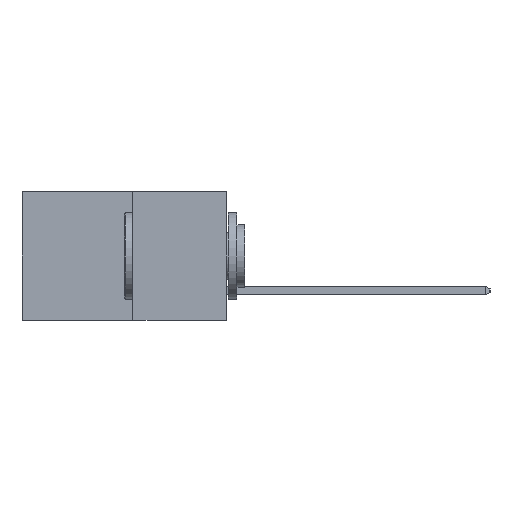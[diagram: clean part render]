
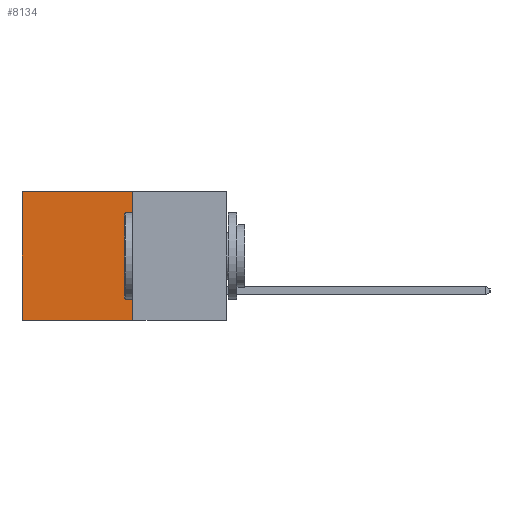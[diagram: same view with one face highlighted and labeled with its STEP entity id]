
A CAD part, left-side view. The second image highlights one B-rep face of the part: STEP entity #8134.
In plain terms, the highlighted planar face has unit normal (-1, 0, 0).
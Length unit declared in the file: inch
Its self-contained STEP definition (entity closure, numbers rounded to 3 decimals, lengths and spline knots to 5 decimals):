
#616 = PLANE ( 'NONE',  #6186 ) ;
#659 = EDGE_CURVE ( 'NONE', #6049, #8187, #4070, .T. ) ;
#682 = CARTESIAN_POINT ( 'NONE',  ( 0.277, 0.59, 0. ) ) ;
#686 = VECTOR ( 'NONE', #6309, 39.37008 ) ;
#1012 = VECTOR ( 'NONE', #6744, 39.37008 ) ;
#1179 = VERTEX_POINT ( 'NONE', #6164 ) ;
#1373 = DIRECTION ( 'NONE',  ( 0., 0., -1. ) ) ;
#1428 = CARTESIAN_POINT ( 'NONE',  ( 0.277, 0.27, -0.37 ) ) ;
#1877 = EDGE_LOOP ( 'NONE', ( #8418, #8705, #6955, #3349 ) ) ;
#2215 = EDGE_CURVE ( 'NONE', #1179, #5717, #4808, .T. ) ;
#2420 = VECTOR ( 'NONE', #3622, 39.37008 ) ;
#2565 = VECTOR ( 'NONE', #4669, 39.37008 ) ;
#3349 = ORIENTED_EDGE ( 'NONE', *, *, #659, .T. ) ;
#3531 = CARTESIAN_POINT ( 'NONE',  ( 0.277, 0.27, -0.37 ) ) ;
#3622 = DIRECTION ( 'NONE',  ( 0., 0., -1. ) ) ;
#4070 = LINE ( 'NONE', #6449, #686 ) ;
#4201 = LINE ( 'NONE', #4583, #2565 ) ;
#4291 = LINE ( 'NONE', #5674, #2420 ) ;
#4583 = CARTESIAN_POINT ( 'NONE',  ( 0.277, 0.27, -0.37 ) ) ;
#4669 = DIRECTION ( 'NONE',  ( 0., 0., -1. ) ) ;
#4808 = LINE ( 'NONE', #1428, #1012 ) ;
#5605 = DIRECTION ( 'NONE',  ( 1., 0., 0. ) ) ;
#5674 = CARTESIAN_POINT ( 'NONE',  ( 0.277, 0.59, -0.37 ) ) ;
#5717 = VERTEX_POINT ( 'NONE', #8842 ) ;
#5873 = CARTESIAN_POINT ( 'NONE',  ( 0.277, 0.27, 0. ) ) ;
#6049 = VERTEX_POINT ( 'NONE', #5873 ) ;
#6164 = CARTESIAN_POINT ( 'NONE',  ( 0.277, 0.27, -0.37 ) ) ;
#6168 = EDGE_CURVE ( 'NONE', #6049, #1179, #4201, .T. ) ;
#6186 = AXIS2_PLACEMENT_3D ( 'NONE', #3531, #5605, #1373 ) ;
#6309 = DIRECTION ( 'NONE',  ( 0., 1., 0. ) ) ;
#6449 = CARTESIAN_POINT ( 'NONE',  ( 0.277, 0.27, 0. ) ) ;
#6744 = DIRECTION ( 'NONE',  ( 0., 1., 0. ) ) ;
#6955 = ORIENTED_EDGE ( 'NONE', *, *, #6168, .F. ) ;
#6998 = FACE_OUTER_BOUND ( 'NONE', #1877, .T. ) ;
#7665 = EDGE_CURVE ( 'NONE', #8187, #5717, #4291, .T. ) ;
#8134 = ADVANCED_FACE ( 'NONE', ( #6998 ), #616, .F. ) ;
#8187 = VERTEX_POINT ( 'NONE', #682 ) ;
#8418 = ORIENTED_EDGE ( 'NONE', *, *, #7665, .T. ) ;
#8705 = ORIENTED_EDGE ( 'NONE', *, *, #2215, .F. ) ;
#8842 = CARTESIAN_POINT ( 'NONE',  ( 0.277, 0.59, -0.37 ) ) ;
